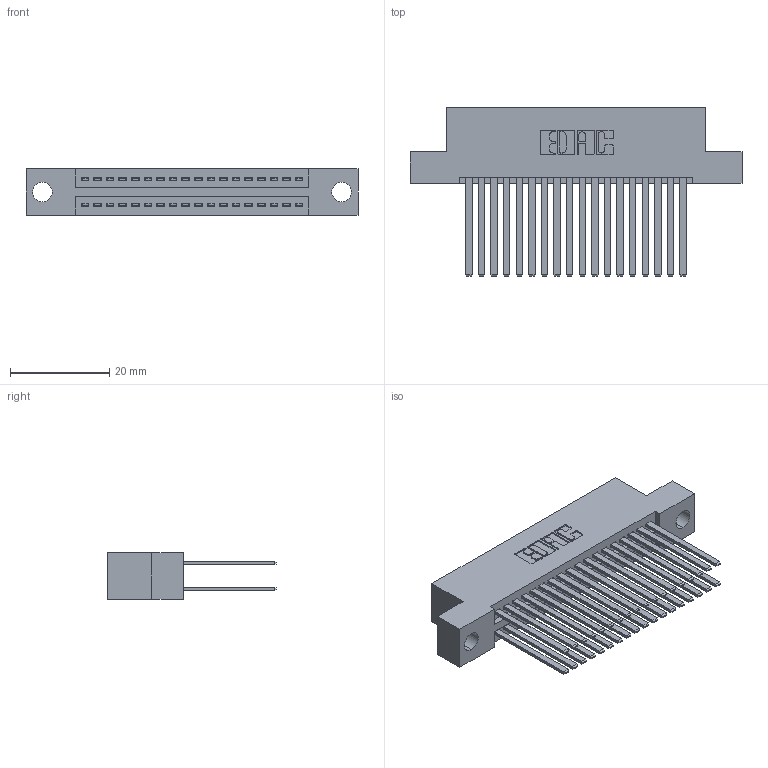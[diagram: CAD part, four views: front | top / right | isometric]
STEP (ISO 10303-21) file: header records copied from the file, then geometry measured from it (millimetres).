
FILE_DESCRIPTION (( 'STEP AP203' ), '1' );
FILE_NAME ('345-036-544-204.STEP', '2018-08-29T23:43:43', ( '' ), ( '' ), 'SwSTEP 2.0', 'SolidWorks 2016', '' );
FILE_SCHEMA (( 'CONFIG_CONTROL_DESIGN' ));
Length unit declared in the file: inch
Products named in the file (3): 345 Part_Flush Mounting Lugs - 0.156 Dia-TH; 345-292-001_345-293-144; 345-036-544-204
Assembly tree (37 placements, depth 2):
  345-036-544-204
    345 Part_Flush Mounting Lugs - 0.156 Dia-TH
    345-292-001_345-293-144  x36
Bounding box: 66.93 x 33.96 x 9.4 mm (x, y, z)
Volume: 6695.6 mm3; surface area: 10726.6 mm2
Topology: 37 solids, 37 shells, 1710 faces, 5057 edges, 3322 vertices
Faces by surface type: plane 1124, cylinder 586
Entity records: 17173 total; most frequent: CARTESIAN_POINT 2900, ORIENTED_EDGE 2834, DIRECTION 2585, EDGE_CURVE 1417, VECTOR 1217, LINE 1217, VERTEX_POINT 942, AXIS2_PLACEMENT_3D 684
